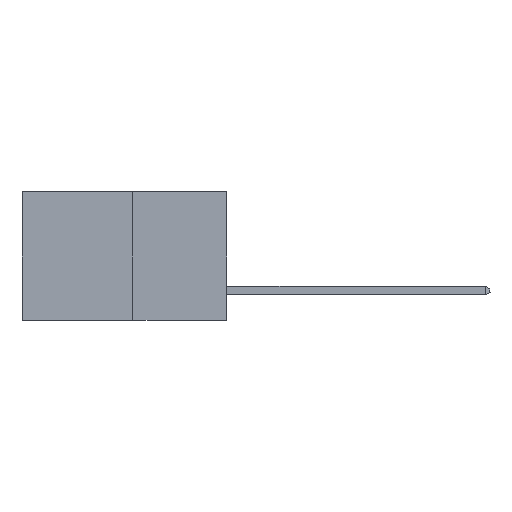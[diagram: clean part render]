
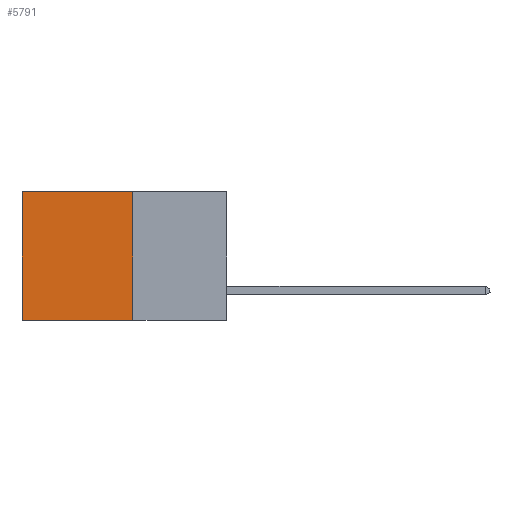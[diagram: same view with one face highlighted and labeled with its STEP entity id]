
A CAD part, left-side view. The second image highlights one B-rep face of the part: STEP entity #5791.
In plain terms, the highlighted planar face has unit normal (-1, 0, 0).
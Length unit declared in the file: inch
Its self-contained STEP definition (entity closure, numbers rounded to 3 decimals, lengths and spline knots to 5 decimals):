
#684 = AXIS2_PLACEMENT_3D ( 'NONE', #13011, #12870, #12731 ) ;
#1338 = DIRECTION ( 'NONE',  ( 0., 0., -1. ) ) ;
#2194 = VERTEX_POINT ( 'NONE', #14376 ) ;
#2305 = VERTEX_POINT ( 'NONE', #22822 ) ;
#2401 = CARTESIAN_POINT ( 'NONE',  ( 0.277, 0.27, 0. ) ) ;
#2963 = ORIENTED_EDGE ( 'NONE', *, *, #16046, .T. ) ;
#3227 = CARTESIAN_POINT ( 'NONE',  ( 0.277, 0.27, -0.37 ) ) ;
#3550 = VECTOR ( 'NONE', #11262, 39.37008 ) ;
#5124 = EDGE_CURVE ( 'NONE', #17003, #2194, #12483, .T. ) ;
#5791 = ADVANCED_FACE ( 'NONE', ( #12159 ), #13983, .F. ) ;
#6512 = VECTOR ( 'NONE', #21980, 39.37008 ) ;
#7507 = EDGE_LOOP ( 'NONE', ( #20659, #10845, #17903, #2963 ) ) ;
#10721 = EDGE_CURVE ( 'NONE', #2305, #13835, #19356, .T. ) ;
#10845 = ORIENTED_EDGE ( 'NONE', *, *, #17569, .F. ) ;
#11262 = DIRECTION ( 'NONE',  ( 0., 0., -1. ) ) ;
#11341 = CARTESIAN_POINT ( 'NONE',  ( 0.277, 0.59, -0.37 ) ) ;
#11566 = VECTOR ( 'NONE', #1338, 39.37008 ) ;
#12086 = CARTESIAN_POINT ( 'NONE',  ( 0.277, 0.27, -0.37 ) ) ;
#12159 = FACE_OUTER_BOUND ( 'NONE', #7507, .T. ) ;
#12483 = LINE ( 'NONE', #11341, #3550 ) ;
#12731 = DIRECTION ( 'NONE',  ( 0., 0., -1. ) ) ;
#12870 = DIRECTION ( 'NONE',  ( 1., 0., 0. ) ) ;
#13011 = CARTESIAN_POINT ( 'NONE',  ( 0.277, 0.27, -0.37 ) ) ;
#13835 = VERTEX_POINT ( 'NONE', #16824 ) ;
#13952 = DIRECTION ( 'NONE',  ( 0., 1., 0. ) ) ;
#13983 = PLANE ( 'NONE',  #684 ) ;
#14202 = CARTESIAN_POINT ( 'NONE',  ( 0.277, 0.59, 0. ) ) ;
#14376 = CARTESIAN_POINT ( 'NONE',  ( 0.277, 0.59, -0.37 ) ) ;
#14552 = VECTOR ( 'NONE', #13952, 39.37008 ) ;
#16046 = EDGE_CURVE ( 'NONE', #2305, #17003, #20673, .T. ) ;
#16824 = CARTESIAN_POINT ( 'NONE',  ( 0.277, 0.27, -0.37 ) ) ;
#17003 = VERTEX_POINT ( 'NONE', #14202 ) ;
#17569 = EDGE_CURVE ( 'NONE', #13835, #2194, #18724, .T. ) ;
#17903 = ORIENTED_EDGE ( 'NONE', *, *, #10721, .F. ) ;
#18724 = LINE ( 'NONE', #3227, #14552 ) ;
#19356 = LINE ( 'NONE', #12086, #11566 ) ;
#20659 = ORIENTED_EDGE ( 'NONE', *, *, #5124, .T. ) ;
#20673 = LINE ( 'NONE', #2401, #6512 ) ;
#21980 = DIRECTION ( 'NONE',  ( 0., 1., 0. ) ) ;
#22822 = CARTESIAN_POINT ( 'NONE',  ( 0.277, 0.27, 0. ) ) ;
